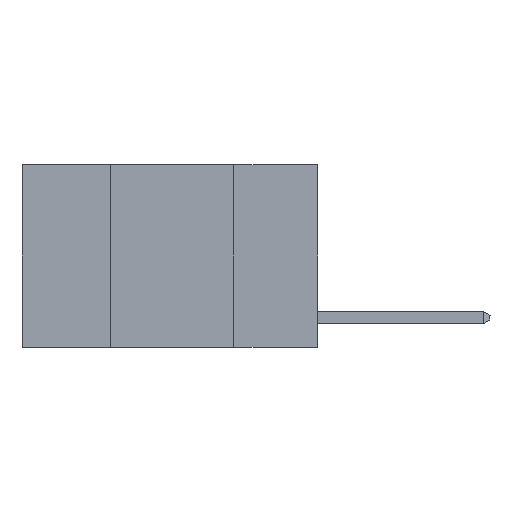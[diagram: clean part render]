
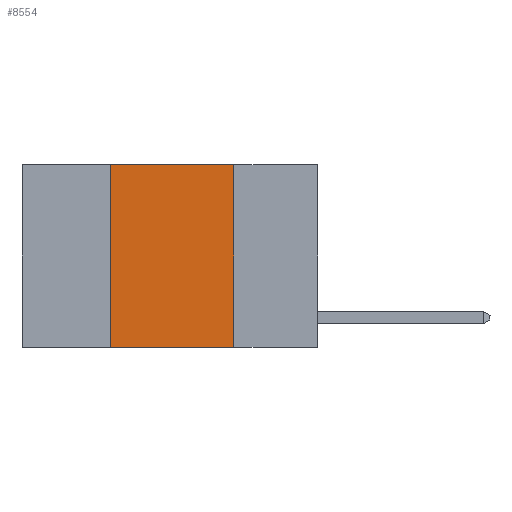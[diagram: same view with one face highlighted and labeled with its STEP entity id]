
A CAD part, left-side view. The second image highlights one B-rep face of the part: STEP entity #8554.
In plain terms, the highlighted planar face has unit normal (-1, 0, 0).
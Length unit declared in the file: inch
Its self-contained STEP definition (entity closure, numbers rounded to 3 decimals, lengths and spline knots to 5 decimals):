
#786 = CARTESIAN_POINT ( 'NONE',  ( 0., 0.42, 0. ) ) ;
#1246 = LINE ( 'NONE', #10229, #16980 ) ;
#1781 = EDGE_CURVE ( 'NONE', #25745, #14985, #13889, .T. ) ;
#2719 = AXIS2_PLACEMENT_3D ( 'NONE', #19991, #24801, #4936 ) ;
#4936 = DIRECTION ( 'NONE',  ( 0., 0., -1. ) ) ;
#5235 = VERTEX_POINT ( 'NONE', #786 ) ;
#5886 = DIRECTION ( 'NONE',  ( 0., -1., 0. ) ) ;
#6082 = EDGE_CURVE ( 'NONE', #9052, #14985, #1246, .T. ) ;
#6826 = FACE_OUTER_BOUND ( 'NONE', #27945, .T. ) ;
#8435 = VECTOR ( 'NONE', #13897, 39.37008 ) ;
#8554 = ADVANCED_FACE ( 'NONE', ( #6826 ), #26971, .F. ) ;
#9052 = VERTEX_POINT ( 'NONE', #26933 ) ;
#10229 = CARTESIAN_POINT ( 'NONE',  ( 0., 0.6, -0.37 ) ) ;
#11725 = CARTESIAN_POINT ( 'NONE',  ( 0., 0.17, -0.37 ) ) ;
#11862 = DIRECTION ( 'NONE',  ( 0., 0., -1. ) ) ;
#12399 = ORIENTED_EDGE ( 'NONE', *, *, #1781, .F. ) ;
#12669 = ORIENTED_EDGE ( 'NONE', *, *, #20860, .F. ) ;
#13605 = CARTESIAN_POINT ( 'NONE',  ( 0., 0.17, 0. ) ) ;
#13889 = LINE ( 'NONE', #13605, #26166 ) ;
#13897 = DIRECTION ( 'NONE',  ( 0., 0., 1. ) ) ;
#14393 = CARTESIAN_POINT ( 'NONE',  ( 0., 0.6, 0. ) ) ;
#14985 = VERTEX_POINT ( 'NONE', #11725 ) ;
#16010 = EDGE_CURVE ( 'NONE', #5235, #25745, #16564, .T. ) ;
#16564 = LINE ( 'NONE', #14393, #24967 ) ;
#16980 = VECTOR ( 'NONE', #5886, 39.37008 ) ;
#17579 = CARTESIAN_POINT ( 'NONE',  ( 0., 0.17, 0. ) ) ;
#17631 = ORIENTED_EDGE ( 'NONE', *, *, #6082, .T. ) ;
#19991 = CARTESIAN_POINT ( 'NONE',  ( 0., 0.6, 0. ) ) ;
#20269 = CARTESIAN_POINT ( 'NONE',  ( 0., 0.42, 0. ) ) ;
#20860 = EDGE_CURVE ( 'NONE', #9052, #5235, #24509, .T. ) ;
#23533 = DIRECTION ( 'NONE',  ( 0., -1., 0. ) ) ;
#24509 = LINE ( 'NONE', #20269, #8435 ) ;
#24801 = DIRECTION ( 'NONE',  ( 1., 0., 0. ) ) ;
#24967 = VECTOR ( 'NONE', #23533, 39.37008 ) ;
#25745 = VERTEX_POINT ( 'NONE', #17579 ) ;
#25832 = ORIENTED_EDGE ( 'NONE', *, *, #16010, .F. ) ;
#26166 = VECTOR ( 'NONE', #11862, 39.37008 ) ;
#26933 = CARTESIAN_POINT ( 'NONE',  ( 0., 0.42, -0.37 ) ) ;
#26971 = PLANE ( 'NONE',  #2719 ) ;
#27945 = EDGE_LOOP ( 'NONE', ( #12399, #25832, #12669, #17631 ) ) ;
